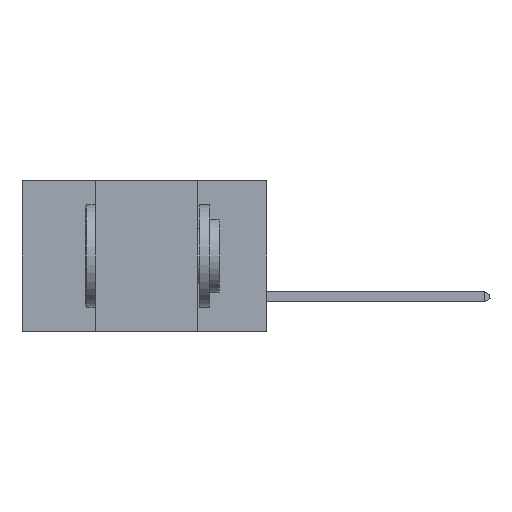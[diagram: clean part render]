
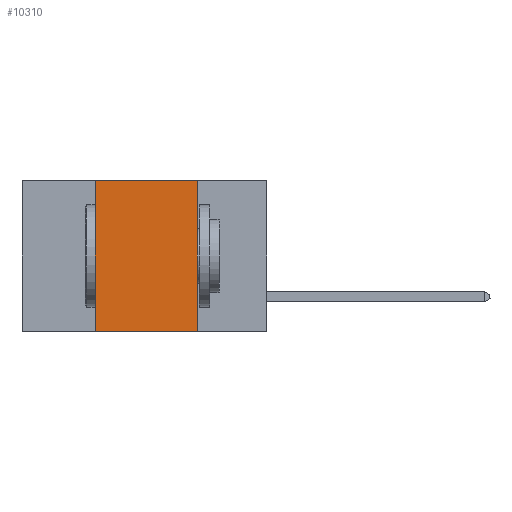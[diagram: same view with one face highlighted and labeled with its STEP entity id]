
A CAD part, left-side view. The second image highlights one B-rep face of the part: STEP entity #10310.
In plain terms, the highlighted planar face has unit normal (-1, 0, 0).
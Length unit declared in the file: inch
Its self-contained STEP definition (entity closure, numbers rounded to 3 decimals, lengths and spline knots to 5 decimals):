
#92 = DIRECTION ( 'NONE',  ( 0., 0., 1. ) ) ;
#126 = DIRECTION ( 'NONE',  ( 0., -1., 0. ) ) ;
#462 = LINE ( 'NONE', #4238, #4482 ) ;
#843 = VERTEX_POINT ( 'NONE', #7454 ) ;
#1699 = EDGE_CURVE ( 'NONE', #3346, #843, #7608, .T. ) ;
#1835 = ORIENTED_EDGE ( 'NONE', *, *, #1699, .F. ) ;
#1871 = LINE ( 'NONE', #11418, #2515 ) ;
#2158 = EDGE_CURVE ( 'NONE', #7823, #10254, #12694, .T. ) ;
#2288 = ORIENTED_EDGE ( 'NONE', *, *, #2158, .T. ) ;
#2388 = AXIS2_PLACEMENT_3D ( 'NONE', #10812, #11809, #2677 ) ;
#2515 = VECTOR ( 'NONE', #4135, 39.37008 ) ;
#2677 = DIRECTION ( 'NONE',  ( 0., 0., -1. ) ) ;
#3294 = DIRECTION ( 'NONE',  ( 0., -1., 0. ) ) ;
#3346 = VERTEX_POINT ( 'NONE', #12823 ) ;
#4135 = DIRECTION ( 'NONE',  ( 0., 0., -1. ) ) ;
#4238 = CARTESIAN_POINT ( 'NONE',  ( 0., 0.42, 0. ) ) ;
#4482 = VECTOR ( 'NONE', #92, 39.37008 ) ;
#4609 = CARTESIAN_POINT ( 'NONE',  ( 0., 0.17, -0.37 ) ) ;
#5369 = CARTESIAN_POINT ( 'NONE',  ( 0., 0.6, -0.37 ) ) ;
#5819 = VECTOR ( 'NONE', #3294, 39.37008 ) ;
#6642 = ORIENTED_EDGE ( 'NONE', *, *, #8890, .F. ) ;
#7454 = CARTESIAN_POINT ( 'NONE',  ( 0., 0.17, 0. ) ) ;
#7608 = LINE ( 'NONE', #10487, #8581 ) ;
#7719 = CARTESIAN_POINT ( 'NONE',  ( 0., 0.42, -0.37 ) ) ;
#7823 = VERTEX_POINT ( 'NONE', #7719 ) ;
#8581 = VECTOR ( 'NONE', #126, 39.37008 ) ;
#8890 = EDGE_CURVE ( 'NONE', #7823, #3346, #462, .T. ) ;
#8927 = EDGE_CURVE ( 'NONE', #843, #10254, #1871, .T. ) ;
#10254 = VERTEX_POINT ( 'NONE', #4609 ) ;
#10310 = ADVANCED_FACE ( 'NONE', ( #11611 ), #12932, .F. ) ;
#10487 = CARTESIAN_POINT ( 'NONE',  ( 0., 0.6, 0. ) ) ;
#10812 = CARTESIAN_POINT ( 'NONE',  ( 0., 0.6, 0. ) ) ;
#11418 = CARTESIAN_POINT ( 'NONE',  ( 0., 0.17, 0. ) ) ;
#11611 = FACE_OUTER_BOUND ( 'NONE', #11752, .T. ) ;
#11752 = EDGE_LOOP ( 'NONE', ( #12679, #1835, #6642, #2288 ) ) ;
#11809 = DIRECTION ( 'NONE',  ( 1., 0., 0. ) ) ;
#12679 = ORIENTED_EDGE ( 'NONE', *, *, #8927, .F. ) ;
#12694 = LINE ( 'NONE', #5369, #5819 ) ;
#12823 = CARTESIAN_POINT ( 'NONE',  ( 0., 0.42, 0. ) ) ;
#12932 = PLANE ( 'NONE',  #2388 ) ;
